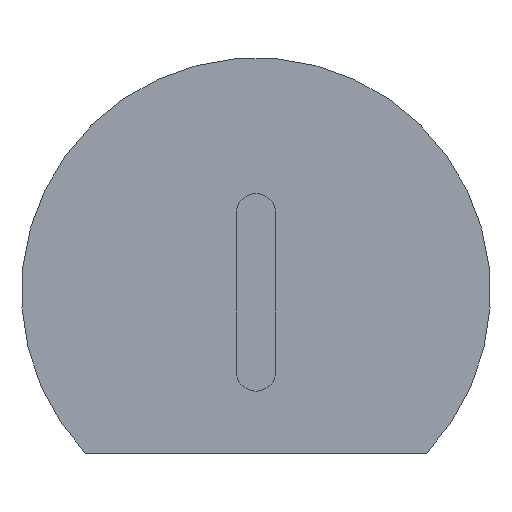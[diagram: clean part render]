
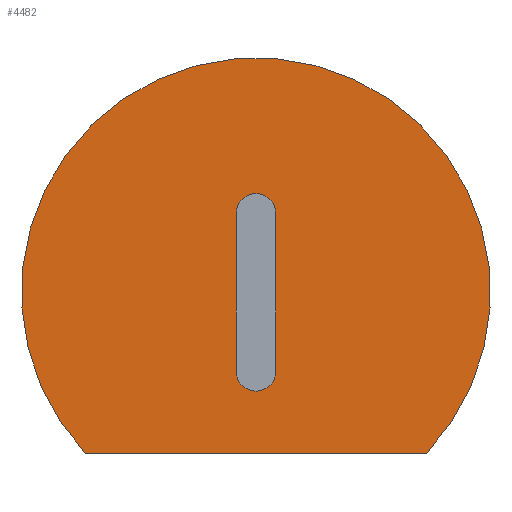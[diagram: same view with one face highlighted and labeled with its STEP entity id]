
A CAD part, left-side view. The second image highlights one B-rep face of the part: STEP entity #4482.
In plain terms, the highlighted planar face has unit normal (-1, 0, 0).
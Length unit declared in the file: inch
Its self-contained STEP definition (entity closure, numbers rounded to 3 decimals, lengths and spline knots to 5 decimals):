
#5 = ORIENTED_EDGE ( 'NONE', *, *, #4537, .T. ) ;
#60 = VECTOR ( 'NONE', #1698, 39.37008 ) ;
#77 = ORIENTED_EDGE ( 'NONE', *, *, #2038, .T. ) ;
#200 = EDGE_CURVE ( 'NONE', #736, #3331, #4116, .T. ) ;
#481 = ORIENTED_EDGE ( 'NONE', *, *, #750, .F. ) ;
#504 = DIRECTION ( 'NONE',  ( 0., 0., -1. ) ) ;
#515 = CARTESIAN_POINT ( 'NONE',  ( -0.52991, 0.51009, -0.04817 ) ) ;
#517 = CARTESIAN_POINT ( 'NONE',  ( -0.52991, 0.51009, -0.12817 ) ) ;
#540 = EDGE_LOOP ( 'NONE', ( #4598, #882, #481, #4527, #4327 ) ) ;
#736 = VERTEX_POINT ( 'NONE', #4132 ) ;
#750 = EDGE_CURVE ( 'NONE', #1789, #2312, #3520, .T. ) ;
#882 = ORIENTED_EDGE ( 'NONE', *, *, #4787, .F. ) ;
#939 = DIRECTION ( 'NONE',  ( 0., 0., -1. ) ) ;
#1036 = CIRCLE ( 'NONE', #3898, 0.02 ) ;
#1171 = AXIS2_PLACEMENT_3D ( 'NONE', #515, #3418, #939 ) ;
#1228 = AXIS2_PLACEMENT_3D ( 'NONE', #1413, #3465, #5189 ) ;
#1235 = CARTESIAN_POINT ( 'NONE',  ( -0.52991, 0.49009, -0.12817 ) ) ;
#1413 = CARTESIAN_POINT ( 'NONE',  ( -0.52991, 0.51009, -0.12817 ) ) ;
#1600 = EDGE_CURVE ( 'NONE', #1783, #1789, #4510, .T. ) ;
#1666 = DIRECTION ( 'NONE',  ( -1., 0., 0. ) ) ;
#1698 = DIRECTION ( 'NONE',  ( 0., 0., 1. ) ) ;
#1783 = VERTEX_POINT ( 'NONE', #1235 ) ;
#1789 = VERTEX_POINT ( 'NONE', #4159 ) ;
#1954 = EDGE_CURVE ( 'NONE', #3331, #1783, #1036, .T. ) ;
#1953 = CARTESIAN_POINT ( 'NONE',  ( -0.52991, 0.53009, 0.03183 ) ) ;
#2038 = EDGE_CURVE ( 'NONE', #5426, #4997, #2282, .T. ) ;
#2113 = DIRECTION ( 'NONE',  ( -1., 0., 0. ) ) ;
#2254 = VECTOR ( 'NONE', #504, 39.37008 ) ;
#2282 = CIRCLE ( 'NONE', #4158, 0.2375 ) ;
#2284 = CARTESIAN_POINT ( 'NONE',  ( -0.52991, 0.51009, -0.14817 ) ) ;
#2312 = VERTEX_POINT ( 'NONE', #1953 ) ;
#2685 = PLANE ( 'NONE',  #1171 ) ;
#2700 = VECTOR ( 'NONE', #5105, 39.37008 ) ;
#2912 = CARTESIAN_POINT ( 'NONE',  ( -0.52991, 0.51009, -0.04817 ) ) ;
#3331 = VERTEX_POINT ( 'NONE', #2284 ) ;
#3350 = DIRECTION ( 'NONE',  ( -1., 0., 0. ) ) ;
#3418 = DIRECTION ( 'NONE',  ( -1., 0., 0. ) ) ;
#3421 = DIRECTION ( 'NONE',  ( 0., 0., -1. ) ) ;
#3465 = DIRECTION ( 'NONE',  ( -1., 0., 0. ) ) ;
#3478 = LINE ( 'NONE', #4275, #2254 ) ;
#3520 = CIRCLE ( 'NONE', #3835, 0.02 ) ;
#3561 = FACE_OUTER_BOUND ( 'NONE', #3589, .T. ) ;
#3589 = EDGE_LOOP ( 'NONE', ( #5, #77 ) ) ;
#3835 = AXIS2_PLACEMENT_3D ( 'NONE', #5007, #2113, #5027 ) ;
#3898 = AXIS2_PLACEMENT_3D ( 'NONE', #517, #3350, #3421 ) ;
#3952 = FACE_BOUND ( 'NONE', #540, .T. ) ;
#4116 = CIRCLE ( 'NONE', #1228, 0.02 ) ;
#4132 = CARTESIAN_POINT ( 'NONE',  ( -0.52991, 0.53009, -0.12817 ) ) ;
#4158 = AXIS2_PLACEMENT_3D ( 'NONE', #2912, #1666, #4569 ) ;
#4159 = CARTESIAN_POINT ( 'NONE',  ( -0.52991, 0.49009, 0.03183 ) ) ;
#4186 = CARTESIAN_POINT ( 'NONE',  ( -0.52991, 0.49009, -0.12817 ) ) ;
#4264 = CARTESIAN_POINT ( 'NONE',  ( -0.52991, 0.68288, -0.21111 ) ) ;
#4275 = CARTESIAN_POINT ( 'NONE',  ( -0.52991, 0.53009, -0.12817 ) ) ;
#4327 = ORIENTED_EDGE ( 'NONE', *, *, #1954, .F. ) ;
#4482 = ADVANCED_FACE ( 'NONE', ( #3952, #3561 ), #2685, .T. ) ;
#4489 = LINE ( 'NONE', #5124, #2700 ) ;
#4510 = LINE ( 'NONE', #4186, #60 ) ;
#4527 = ORIENTED_EDGE ( 'NONE', *, *, #1600, .F. ) ;
#4537 = EDGE_CURVE ( 'NONE', #4997, #5426, #4489, .T. ) ;
#4569 = DIRECTION ( 'NONE',  ( 0., 0., -1. ) ) ;
#4598 = ORIENTED_EDGE ( 'NONE', *, *, #200, .F. ) ;
#4787 = EDGE_CURVE ( 'NONE', #2312, #736, #3478, .T. ) ;
#4997 = VERTEX_POINT ( 'NONE', #4264 ) ;
#5007 = CARTESIAN_POINT ( 'NONE',  ( -0.52991, 0.51009, 0.03183 ) ) ;
#5027 = DIRECTION ( 'NONE',  ( 0., 0., -1. ) ) ;
#5105 = DIRECTION ( 'NONE',  ( 0., -1., 0. ) ) ;
#5112 = CARTESIAN_POINT ( 'NONE',  ( -0.52991, 0.3373, -0.21111 ) ) ;
#5124 = CARTESIAN_POINT ( 'NONE',  ( -0.52991, 0.26009, -0.21111 ) ) ;
#5189 = DIRECTION ( 'NONE',  ( 0., 0., -1. ) ) ;
#5426 = VERTEX_POINT ( 'NONE', #5112 ) ;
